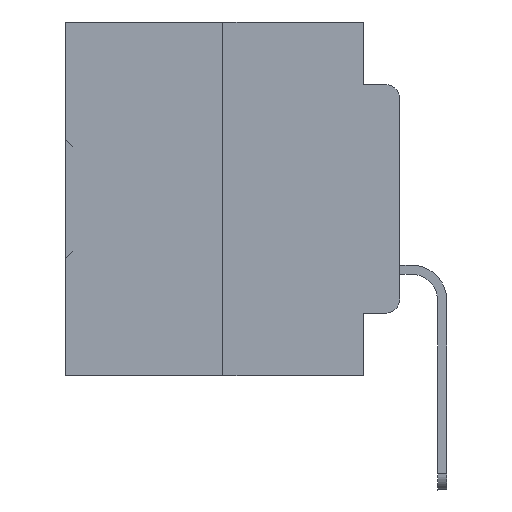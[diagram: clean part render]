
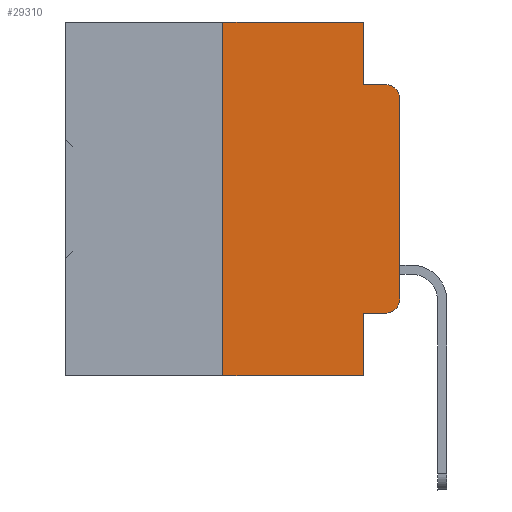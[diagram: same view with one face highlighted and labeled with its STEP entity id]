
A CAD part, left-side view. The second image highlights one B-rep face of the part: STEP entity #29310.
In plain terms, the highlighted planar face has unit normal (-1, 0, 0).
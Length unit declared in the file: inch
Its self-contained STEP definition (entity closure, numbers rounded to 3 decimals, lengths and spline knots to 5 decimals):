
#234 = CARTESIAN_POINT ( 'NONE',  ( 0., 0.051, -0.5 ) ) ;
#400 = VECTOR ( 'NONE', #23128, 39.37008 ) ;
#1424 = EDGE_CURVE ( 'NONE', #6887, #3526, #32773, .T. ) ;
#1726 = EDGE_CURVE ( 'NONE', #24283, #5849, #3301, .T. ) ;
#2141 = CARTESIAN_POINT ( 'NONE',  ( 0., 0.02, -0.3915 ) ) ;
#2330 = FACE_OUTER_BOUND ( 'NONE', #33296, .T. ) ;
#2658 = CARTESIAN_POINT ( 'NONE',  ( 0., 0.473, -0.5 ) ) ;
#2953 = CARTESIAN_POINT ( 'NONE',  ( 0., 0.051, -0.0885 ) ) ;
#3301 = LINE ( 'NONE', #26732, #32461 ) ;
#3526 = VERTEX_POINT ( 'NONE', #24759 ) ;
#4237 = VECTOR ( 'NONE', #13475, 39.37008 ) ;
#4701 = EDGE_CURVE ( 'NONE', #5849, #10833, #16000, .T. ) ;
#5740 = CARTESIAN_POINT ( 'NONE',  ( 0., 0.051, 0. ) ) ;
#5849 = VERTEX_POINT ( 'NONE', #29674 ) ;
#6014 = ORIENTED_EDGE ( 'NONE', *, *, #33071, .F. ) ;
#6241 = EDGE_CURVE ( 'NONE', #35573, #19765, #36328, .T. ) ;
#6364 = DIRECTION ( 'NONE',  ( -1., 0., 0. ) ) ;
#6465 = CARTESIAN_POINT ( 'NONE',  ( 0., 0.25, 0. ) ) ;
#6887 = VERTEX_POINT ( 'NONE', #34130 ) ;
#7495 = ORIENTED_EDGE ( 'NONE', *, *, #25202, .F. ) ;
#8825 = CARTESIAN_POINT ( 'NONE',  ( 0., 0.02, -0.0885 ) ) ;
#9262 = VERTEX_POINT ( 'NONE', #31733 ) ;
#9377 = LINE ( 'NONE', #2658, #16343 ) ;
#9686 = CARTESIAN_POINT ( 'NONE',  ( 0., 0.02, -0.4115 ) ) ;
#10057 = EDGE_CURVE ( 'NONE', #9262, #32051, #28946, .T. ) ;
#10283 = VECTOR ( 'NONE', #34913, 39.37008 ) ;
#10833 = VERTEX_POINT ( 'NONE', #8825 ) ;
#11379 = AXIS2_PLACEMENT_3D ( 'NONE', #2141, #34454, #20233 ) ;
#11874 = LINE ( 'NONE', #5740, #4237 ) ;
#12156 = EDGE_CURVE ( 'NONE', #32051, #24283, #21195, .T. ) ;
#12249 = DIRECTION ( 'NONE',  ( 0., 0., 1. ) ) ;
#12829 = VERTEX_POINT ( 'NONE', #234 ) ;
#13475 = DIRECTION ( 'NONE',  ( 0., 0., -1. ) ) ;
#14959 = DIRECTION ( 'NONE',  ( 0., -1., 0. ) ) ;
#16000 = CIRCLE ( 'NONE', #37485, 0.02 ) ;
#16343 = VECTOR ( 'NONE', #14959, 39.37008 ) ;
#16933 = PLANE ( 'NONE',  #24376 ) ;
#17049 = CARTESIAN_POINT ( 'NONE',  ( 0., 0.051, -0.4115 ) ) ;
#17063 = ORIENTED_EDGE ( 'NONE', *, *, #10057, .T. ) ;
#19765 = VERTEX_POINT ( 'NONE', #2953 ) ;
#20233 = DIRECTION ( 'NONE',  ( 0., 0., -1. ) ) ;
#20289 = LINE ( 'NONE', #34886, #34366 ) ;
#21195 = CIRCLE ( 'NONE', #11379, 0.02 ) ;
#21569 = CARTESIAN_POINT ( 'NONE',  ( 0., 0., -0.3915 ) ) ;
#23128 = DIRECTION ( 'NONE',  ( 0., -1., 0. ) ) ;
#24283 = VERTEX_POINT ( 'NONE', #21569 ) ;
#24376 = AXIS2_PLACEMENT_3D ( 'NONE', #37326, #37519, #28634 ) ;
#24577 = VECTOR ( 'NONE', #30174, 39.37008 ) ;
#24759 = CARTESIAN_POINT ( 'NONE',  ( 0., 0.25, 0. ) ) ;
#25202 = EDGE_CURVE ( 'NONE', #3526, #35573, #37747, .T. ) ;
#25864 = ORIENTED_EDGE ( 'NONE', *, *, #35005, .T. ) ;
#26347 = VECTOR ( 'NONE', #12249, 39.37008 ) ;
#26732 = CARTESIAN_POINT ( 'NONE',  ( 0., 0., 0. ) ) ;
#27045 = ORIENTED_EDGE ( 'NONE', *, *, #1726, .T. ) ;
#27305 = DIRECTION ( 'NONE',  ( 0., 0., 1. ) ) ;
#27824 = ORIENTED_EDGE ( 'NONE', *, *, #1424, .F. ) ;
#28180 = ORIENTED_EDGE ( 'NONE', *, *, #4701, .T. ) ;
#28634 = DIRECTION ( 'NONE',  ( 0., 0., -1. ) ) ;
#28720 = DIRECTION ( 'NONE',  ( 0., -1., 0. ) ) ;
#28946 = LINE ( 'NONE', #17049, #10283 ) ;
#29310 = ADVANCED_FACE ( 'NONE', ( #2330 ), #16933, .F. ) ;
#29674 = CARTESIAN_POINT ( 'NONE',  ( 0., 0., -0.1085 ) ) ;
#29765 = DIRECTION ( 'NONE',  ( 0., 0., -1. ) ) ;
#30174 = DIRECTION ( 'NONE',  ( 0., 0., -1. ) ) ;
#30539 = CARTESIAN_POINT ( 'NONE',  ( 0., 0.051, 0. ) ) ;
#30941 = CARTESIAN_POINT ( 'NONE',  ( 0., 0.051, 0. ) ) ;
#31733 = CARTESIAN_POINT ( 'NONE',  ( 0., 0.051, -0.4115 ) ) ;
#32051 = VERTEX_POINT ( 'NONE', #9686 ) ;
#32165 = CARTESIAN_POINT ( 'NONE',  ( 0., 0.473, 0. ) ) ;
#32461 = VECTOR ( 'NONE', #27305, 39.37008 ) ;
#32773 = LINE ( 'NONE', #6465, #26347 ) ;
#33071 = EDGE_CURVE ( 'NONE', #9262, #12829, #11874, .T. ) ;
#33296 = EDGE_LOOP ( 'NONE', ( #27045, #28180, #35357, #34128, #7495, #27824, #25864, #6014, #17063, #37476 ) ) ;
#33464 = EDGE_CURVE ( 'NONE', #19765, #10833, #20289, .T. ) ;
#34128 = ORIENTED_EDGE ( 'NONE', *, *, #6241, .F. ) ;
#34130 = CARTESIAN_POINT ( 'NONE',  ( 0., 0.25, -0.5 ) ) ;
#34366 = VECTOR ( 'NONE', #28720, 39.37008 ) ;
#34454 = DIRECTION ( 'NONE',  ( -1., 0., 0. ) ) ;
#34886 = CARTESIAN_POINT ( 'NONE',  ( 0., 0.051, -0.0885 ) ) ;
#34913 = DIRECTION ( 'NONE',  ( 0., -1., 0. ) ) ;
#35005 = EDGE_CURVE ( 'NONE', #6887, #12829, #9377, .T. ) ;
#35357 = ORIENTED_EDGE ( 'NONE', *, *, #33464, .F. ) ;
#35573 = VERTEX_POINT ( 'NONE', #30941 ) ;
#36328 = LINE ( 'NONE', #30539, #24577 ) ;
#37326 = CARTESIAN_POINT ( 'NONE',  ( 0., 0.473, 0. ) ) ;
#37476 = ORIENTED_EDGE ( 'NONE', *, *, #12156, .T. ) ;
#37485 = AXIS2_PLACEMENT_3D ( 'NONE', #37877, #6364, #29765 ) ;
#37519 = DIRECTION ( 'NONE',  ( 1., 0., 0. ) ) ;
#37747 = LINE ( 'NONE', #32165, #400 ) ;
#37877 = CARTESIAN_POINT ( 'NONE',  ( 0., 0.02, -0.1085 ) ) ;
